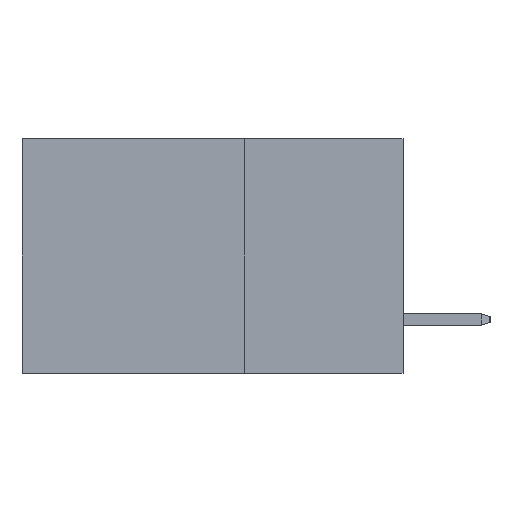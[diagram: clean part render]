
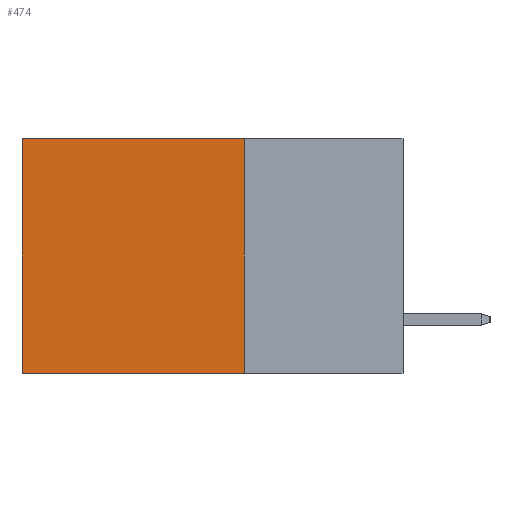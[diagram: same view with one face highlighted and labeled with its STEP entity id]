
A CAD part, left-side view. The second image highlights one B-rep face of the part: STEP entity #474.
In plain terms, the highlighted planar face has unit normal (-1, 0, 0).
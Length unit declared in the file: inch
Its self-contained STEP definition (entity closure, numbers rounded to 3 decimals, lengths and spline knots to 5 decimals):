
#456 = PLANE ( 'NONE',  #736 ) ;
#474 = ADVANCED_FACE ( 'NONE', ( #11519 ), #456, .F. ) ;
#736 = AXIS2_PLACEMENT_3D ( 'NONE', #1967, #3984, #13911 ) ;
#1967 = CARTESIAN_POINT ( 'NONE',  ( 0.2875, 0.25, 0. ) ) ;
#2224 = ORIENTED_EDGE ( 'NONE', *, *, #23434, .T. ) ;
#3016 = CARTESIAN_POINT ( 'NONE',  ( 0.2875, 0.25, 0. ) ) ;
#3693 = CARTESIAN_POINT ( 'NONE',  ( 0.2875, 0.25, -0.37 ) ) ;
#3984 = DIRECTION ( 'NONE',  ( 1., 0., 0. ) ) ;
#4842 = DIRECTION ( 'NONE',  ( 0., 0., -1. ) ) ;
#5247 = LINE ( 'NONE', #14555, #17733 ) ;
#6038 = VERTEX_POINT ( 'NONE', #8909 ) ;
#6171 = VECTOR ( 'NONE', #18497, 39.37008 ) ;
#6617 = ORIENTED_EDGE ( 'NONE', *, *, #11850, .F. ) ;
#6857 = CARTESIAN_POINT ( 'NONE',  ( 0.2875, 0.6, 0. ) ) ;
#7008 = DIRECTION ( 'NONE',  ( 0., 1., 0. ) ) ;
#8274 = EDGE_LOOP ( 'NONE', ( #2224, #13750, #6617, #18962 ) ) ;
#8909 = CARTESIAN_POINT ( 'NONE',  ( 0.2875, 0.25, 0. ) ) ;
#9611 = DIRECTION ( 'NONE',  ( 0., 1., 0. ) ) ;
#10747 = VECTOR ( 'NONE', #4842, 39.37008 ) ;
#11244 = VERTEX_POINT ( 'NONE', #18114 ) ;
#11519 = FACE_OUTER_BOUND ( 'NONE', #8274, .T. ) ;
#11850 = EDGE_CURVE ( 'NONE', #6038, #16502, #12576, .T. ) ;
#12576 = LINE ( 'NONE', #3016, #6171 ) ;
#13249 = LINE ( 'NONE', #3693, #21252 ) ;
#13750 = ORIENTED_EDGE ( 'NONE', *, *, #24337, .F. ) ;
#13911 = DIRECTION ( 'NONE',  ( 0., 0., -1. ) ) ;
#14555 = CARTESIAN_POINT ( 'NONE',  ( 0.2875, 0.25, 0. ) ) ;
#16502 = VERTEX_POINT ( 'NONE', #21005 ) ;
#17733 = VECTOR ( 'NONE', #7008, 39.37008 ) ;
#17918 = LINE ( 'NONE', #6857, #10747 ) ;
#18045 = EDGE_CURVE ( 'NONE', #6038, #23364, #5247, .T. ) ;
#18114 = CARTESIAN_POINT ( 'NONE',  ( 0.2875, 0.6, -0.37 ) ) ;
#18497 = DIRECTION ( 'NONE',  ( 0., 0., -1. ) ) ;
#18962 = ORIENTED_EDGE ( 'NONE', *, *, #18045, .T. ) ;
#19935 = CARTESIAN_POINT ( 'NONE',  ( 0.2875, 0.6, 0. ) ) ;
#21005 = CARTESIAN_POINT ( 'NONE',  ( 0.2875, 0.25, -0.37 ) ) ;
#21252 = VECTOR ( 'NONE', #9611, 39.37008 ) ;
#23364 = VERTEX_POINT ( 'NONE', #19935 ) ;
#23434 = EDGE_CURVE ( 'NONE', #23364, #11244, #17918, .T. ) ;
#24337 = EDGE_CURVE ( 'NONE', #16502, #11244, #13249, .T. ) ;
